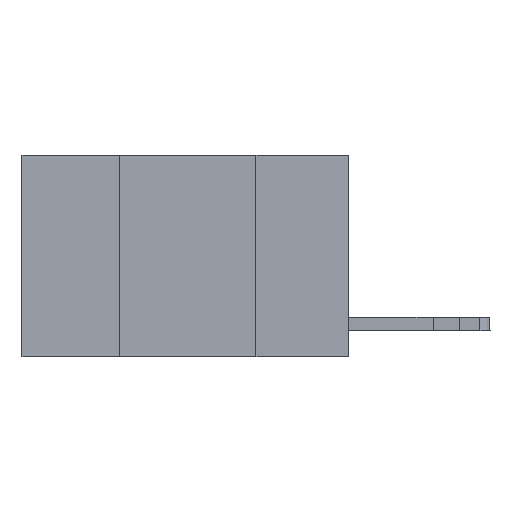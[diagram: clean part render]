
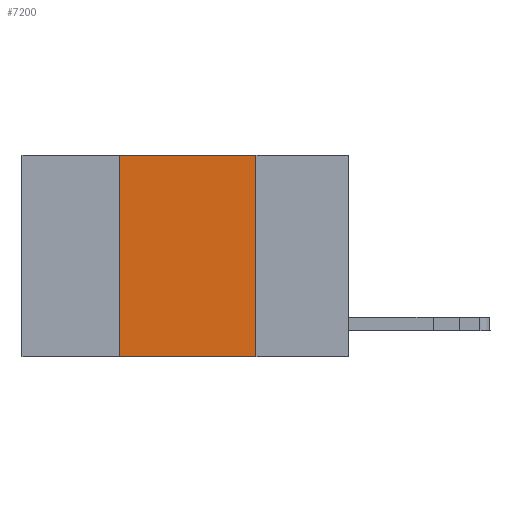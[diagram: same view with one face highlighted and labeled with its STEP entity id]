
A CAD part, left-side view. The second image highlights one B-rep face of the part: STEP entity #7200.
In plain terms, the highlighted planar face has unit normal (-1, 0, 0).
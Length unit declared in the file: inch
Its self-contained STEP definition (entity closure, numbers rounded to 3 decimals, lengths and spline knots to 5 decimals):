
#245 = LINE ( 'NONE', #8408, #20535 ) ;
#1669 = CARTESIAN_POINT ( 'NONE',  ( 0., 0.17, 0. ) ) ;
#2416 = LINE ( 'NONE', #20692, #4170 ) ;
#3417 = LINE ( 'NONE', #1669, #20533 ) ;
#4030 = VERTEX_POINT ( 'NONE', #9598 ) ;
#4170 = VECTOR ( 'NONE', #8187, 39.37008 ) ;
#5149 = DIRECTION ( 'NONE',  ( 0., -1., 0. ) ) ;
#5174 = VERTEX_POINT ( 'NONE', #18346 ) ;
#6900 = CARTESIAN_POINT ( 'NONE',  ( 0., 0.6, -0.37 ) ) ;
#7009 = ORIENTED_EDGE ( 'NONE', *, *, #13556, .F. ) ;
#7200 = ADVANCED_FACE ( 'NONE', ( #8946 ), #23326, .F. ) ;
#7907 = CARTESIAN_POINT ( 'NONE',  ( 0., 0.42, 0. ) ) ;
#8187 = DIRECTION ( 'NONE',  ( 0., 0., 1. ) ) ;
#8408 = CARTESIAN_POINT ( 'NONE',  ( 0., 0.6, 0. ) ) ;
#8946 = FACE_OUTER_BOUND ( 'NONE', #16698, .T. ) ;
#9598 = CARTESIAN_POINT ( 'NONE',  ( 0., 0.42, -0.37 ) ) ;
#10742 = EDGE_CURVE ( 'NONE', #4030, #16450, #16951, .T. ) ;
#11349 = ORIENTED_EDGE ( 'NONE', *, *, #10742, .T. ) ;
#13074 = CARTESIAN_POINT ( 'NONE',  ( 0., 0.6, 0. ) ) ;
#13443 = VERTEX_POINT ( 'NONE', #7907 ) ;
#13556 = EDGE_CURVE ( 'NONE', #4030, #13443, #2416, .T. ) ;
#14603 = EDGE_CURVE ( 'NONE', #13443, #5174, #245, .T. ) ;
#15093 = DIRECTION ( 'NONE',  ( 0., -1., 0. ) ) ;
#15614 = DIRECTION ( 'NONE',  ( 0., 0., -1. ) ) ;
#15623 = DIRECTION ( 'NONE',  ( 1., 0., 0. ) ) ;
#16450 = VERTEX_POINT ( 'NONE', #20044 ) ;
#16698 = EDGE_LOOP ( 'NONE', ( #25321, #24337, #7009, #11349 ) ) ;
#16951 = LINE ( 'NONE', #6900, #23719 ) ;
#17655 = DIRECTION ( 'NONE',  ( 0., 0., -1. ) ) ;
#18346 = CARTESIAN_POINT ( 'NONE',  ( 0., 0.17, 0. ) ) ;
#20044 = CARTESIAN_POINT ( 'NONE',  ( 0., 0.17, -0.37 ) ) ;
#20533 = VECTOR ( 'NONE', #15614, 39.37008 ) ;
#20535 = VECTOR ( 'NONE', #5149, 39.37008 ) ;
#20692 = CARTESIAN_POINT ( 'NONE',  ( 0., 0.42, 0. ) ) ;
#23326 = PLANE ( 'NONE',  #26229 ) ;
#23719 = VECTOR ( 'NONE', #15093, 39.37008 ) ;
#24337 = ORIENTED_EDGE ( 'NONE', *, *, #14603, .F. ) ;
#25321 = ORIENTED_EDGE ( 'NONE', *, *, #25604, .F. ) ;
#25604 = EDGE_CURVE ( 'NONE', #5174, #16450, #3417, .T. ) ;
#26229 = AXIS2_PLACEMENT_3D ( 'NONE', #13074, #15623, #17655 ) ;
